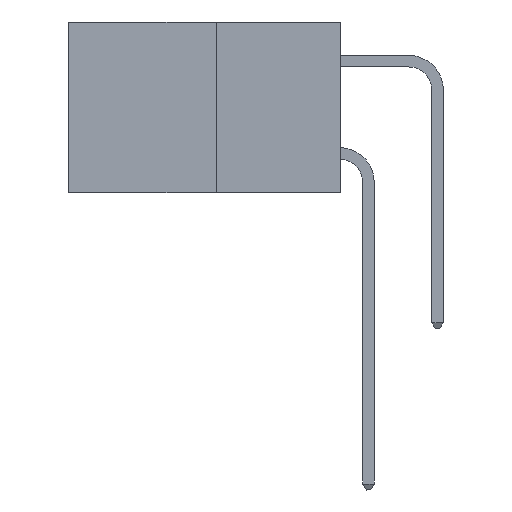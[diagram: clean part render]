
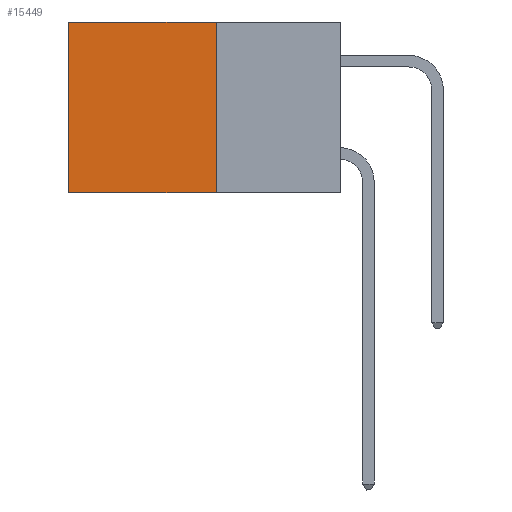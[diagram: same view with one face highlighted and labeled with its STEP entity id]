
A CAD part, left-side view. The second image highlights one B-rep face of the part: STEP entity #15449.
In plain terms, the highlighted planar face has unit normal (-1, 0, 0).
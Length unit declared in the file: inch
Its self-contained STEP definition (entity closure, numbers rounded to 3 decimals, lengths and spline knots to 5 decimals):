
#445 = VERTEX_POINT ( 'NONE', #9784 ) ;
#566 = EDGE_CURVE ( 'NONE', #2838, #15706, #15194, .T. ) ;
#2345 = CARTESIAN_POINT ( 'NONE',  ( 0.277, 0.27, -0.37 ) ) ;
#2507 = EDGE_CURVE ( 'NONE', #15706, #445, #2718, .T. ) ;
#2705 = ORIENTED_EDGE ( 'NONE', *, *, #16657, .T. ) ;
#2718 = LINE ( 'NONE', #12596, #11067 ) ;
#2838 = VERTEX_POINT ( 'NONE', #7678 ) ;
#3448 = VERTEX_POINT ( 'NONE', #18802 ) ;
#3689 = EDGE_CURVE ( 'NONE', #3448, #445, #10276, .T. ) ;
#4088 = DIRECTION ( 'NONE',  ( 0., 0., -1. ) ) ;
#4624 = LINE ( 'NONE', #14193, #13230 ) ;
#5212 = FACE_OUTER_BOUND ( 'NONE', #10138, .T. ) ;
#6560 = AXIS2_PLACEMENT_3D ( 'NONE', #2345, #13764, #4088 ) ;
#7088 = ORIENTED_EDGE ( 'NONE', *, *, #3689, .T. ) ;
#7609 = ORIENTED_EDGE ( 'NONE', *, *, #2507, .F. ) ;
#7678 = CARTESIAN_POINT ( 'NONE',  ( 0.277, 0.27, 0. ) ) ;
#8058 = DIRECTION ( 'NONE',  ( 0., 1., 0. ) ) ;
#9562 = CARTESIAN_POINT ( 'NONE',  ( 0.277, 0.27, -0.37 ) ) ;
#9784 = CARTESIAN_POINT ( 'NONE',  ( 0.277, 0.59, -0.37 ) ) ;
#10138 = EDGE_LOOP ( 'NONE', ( #7088, #7609, #19427, #2705 ) ) ;
#10276 = LINE ( 'NONE', #18055, #18719 ) ;
#10891 = DIRECTION ( 'NONE',  ( 0., 0., -1. ) ) ;
#11067 = VECTOR ( 'NONE', #8058, 39.37008 ) ;
#12596 = CARTESIAN_POINT ( 'NONE',  ( 0.277, 0.27, -0.37 ) ) ;
#13230 = VECTOR ( 'NONE', #17192, 39.37008 ) ;
#13764 = DIRECTION ( 'NONE',  ( 1., 0., 0. ) ) ;
#14193 = CARTESIAN_POINT ( 'NONE',  ( 0.277, 0.27, 0. ) ) ;
#14732 = VECTOR ( 'NONE', #10891, 39.37008 ) ;
#15194 = LINE ( 'NONE', #16162, #14732 ) ;
#15449 = ADVANCED_FACE ( 'NONE', ( #5212 ), #18172, .F. ) ;
#15706 = VERTEX_POINT ( 'NONE', #9562 ) ;
#16162 = CARTESIAN_POINT ( 'NONE',  ( 0.277, 0.27, -0.37 ) ) ;
#16657 = EDGE_CURVE ( 'NONE', #2838, #3448, #4624, .T. ) ;
#17192 = DIRECTION ( 'NONE',  ( 0., 1., 0. ) ) ;
#18055 = CARTESIAN_POINT ( 'NONE',  ( 0.277, 0.59, -0.37 ) ) ;
#18084 = DIRECTION ( 'NONE',  ( 0., 0., -1. ) ) ;
#18172 = PLANE ( 'NONE',  #6560 ) ;
#18719 = VECTOR ( 'NONE', #18084, 39.37008 ) ;
#18802 = CARTESIAN_POINT ( 'NONE',  ( 0.277, 0.59, 0. ) ) ;
#19427 = ORIENTED_EDGE ( 'NONE', *, *, #566, .F. ) ;
